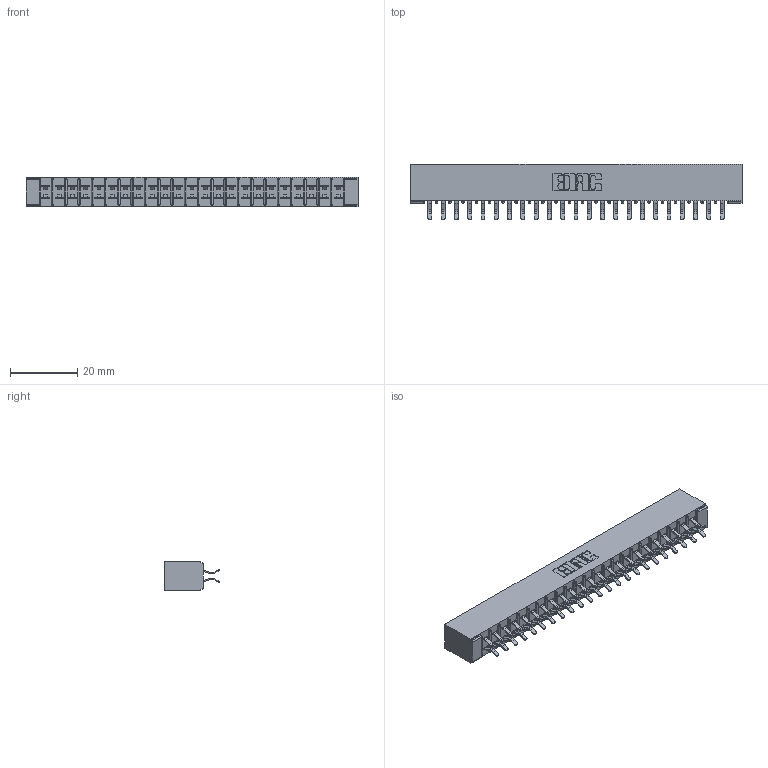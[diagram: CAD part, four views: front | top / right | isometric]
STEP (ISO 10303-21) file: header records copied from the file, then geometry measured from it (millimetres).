
FILE_DESCRIPTION (( 'STEP AP203' ), '1' );
FILE_NAME ('355-046-556-201.STEP', '2019-09-11T14:54:29', ( '' ), ( '' ), 'SwSTEP 2.0', 'SolidWorks 2016', '' );
FILE_SCHEMA (( 'CONFIG_CONTROL_DESIGN' ));
Length unit declared in the file: inch
Products named in the file (3): 305 Part_No Mounting; 355-046-556-201; 305-290-001_556
Assembly tree (47 placements, depth 2):
  355-046-556-201
    305 Part_No Mounting
    305-290-001_556  x46
Bounding box: 99.01 x 16.64 x 8.71 mm (x, y, z)
Volume: 6387.8 mm3; surface area: 12713.8 mm2
Topology: 47 solids, 47 shells, 2684 faces, 7721 edges, 5022 vertices
Faces by surface type: plane 1490, cylinder 1102, sphere 92
Entity records: 27160 total; most frequent: CARTESIAN_POINT 4495, ORIENTED_EDGE 4458, DIRECTION 4365, EDGE_CURVE 2229, LINE 1781, VECTOR 1781, VERTEX_POINT 1422, AXIS2_PLACEMENT_3D 1292
